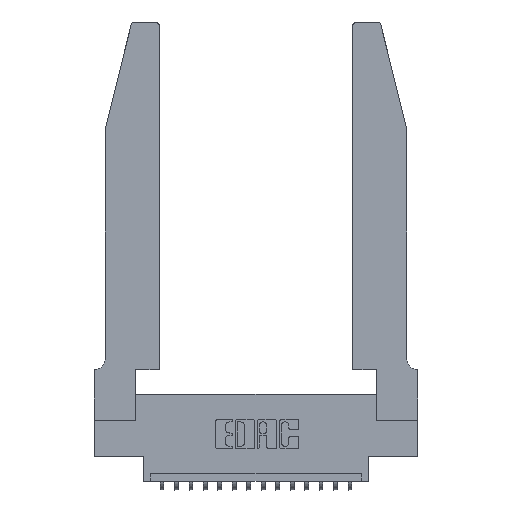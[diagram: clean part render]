
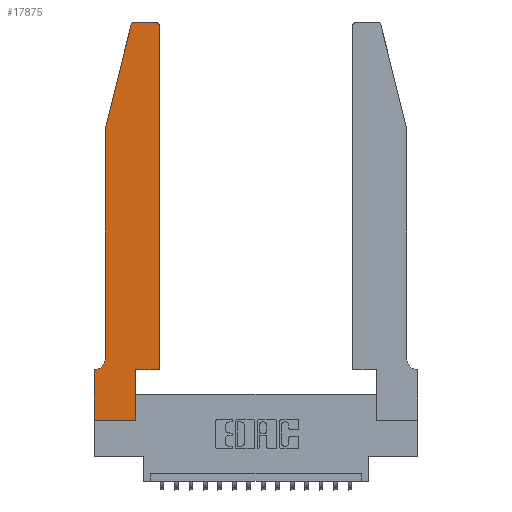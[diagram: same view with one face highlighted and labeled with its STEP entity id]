
A CAD part, top view. The second image highlights one B-rep face of the part: STEP entity #17875.
In plain terms, the highlighted planar face has unit normal (0, 0, 1).
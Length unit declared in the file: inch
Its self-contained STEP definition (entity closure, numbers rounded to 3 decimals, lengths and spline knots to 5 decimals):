
#250 = CARTESIAN_POINT ( 'NONE',  ( 0.0755, 0.35, 0.37 ) ) ;
#420 = CARTESIAN_POINT ( 'NONE',  ( 0.4505, 2.72, 0.37 ) ) ;
#478 = LINE ( 'NONE', #10517, #9352 ) ;
#524 = CARTESIAN_POINT ( 'NONE',  ( 0., 0.35, 0.37 ) ) ;
#538 = CARTESIAN_POINT ( 'NONE',  ( 0.25487, 2.72718, 0.37 ) ) ;
#930 = CARTESIAN_POINT ( 'NONE',  ( 0.0755, 2., 0.37 ) ) ;
#1041 = VECTOR ( 'NONE', #11612, 39.37008 ) ;
#2161 = CARTESIAN_POINT ( 'NONE',  ( 0.0755, 0.42, 0.37 ) ) ;
#2269 = DIRECTION ( 'NONE',  ( 1., 0., 0. ) ) ;
#2365 = EDGE_LOOP ( 'NONE', ( #7171, #6039, #3279, #11034, #11916, #15644, #4440, #10279, #8576, #5864, #8423, #12303 ) ) ;
#2465 = LINE ( 'NONE', #15607, #2705 ) ;
#2705 = VECTOR ( 'NONE', #3567, 39.37008 ) ;
#2795 = LINE ( 'NONE', #14105, #6289 ) ;
#3279 = ORIENTED_EDGE ( 'NONE', *, *, #13928, .T. ) ;
#3567 = DIRECTION ( 'NONE',  ( 1., 0., 0. ) ) ;
#3716 = VERTEX_POINT ( 'NONE', #5914 ) ;
#4440 = ORIENTED_EDGE ( 'NONE', *, *, #6249, .T. ) ;
#5052 = DIRECTION ( 'NONE',  ( 1., 0., 0. ) ) ;
#5201 = DIRECTION ( 'NONE',  ( 0., 0., -1. ) ) ;
#5593 = VERTEX_POINT ( 'NONE', #18524 ) ;
#5864 = ORIENTED_EDGE ( 'NONE', *, *, #7411, .T. ) ;
#5914 = CARTESIAN_POINT ( 'NONE',  ( 0.2865, 0., 0.37 ) ) ;
#5917 = CIRCLE ( 'NONE', #7857, 0.07 ) ;
#5996 = EDGE_CURVE ( 'NONE', #3716, #10725, #478, .T. ) ;
#6039 = ORIENTED_EDGE ( 'NONE', *, *, #7348, .T. ) ;
#6249 = EDGE_CURVE ( 'NONE', #5593, #18419, #2795, .T. ) ;
#6289 = VECTOR ( 'NONE', #17297, 39.37008 ) ;
#6533 = LINE ( 'NONE', #250, #9564 ) ;
#6800 = DIRECTION ( 'NONE',  ( 1., 0., 0. ) ) ;
#7103 = VERTEX_POINT ( 'NONE', #2161 ) ;
#7171 = ORIENTED_EDGE ( 'NONE', *, *, #7546, .T. ) ;
#7348 = EDGE_CURVE ( 'NONE', #12134, #17519, #15580, .T. ) ;
#7411 = EDGE_CURVE ( 'NONE', #10725, #18413, #12380, .T. ) ;
#7546 = EDGE_CURVE ( 'NONE', #13530, #12134, #13526, .T. ) ;
#7550 = CARTESIAN_POINT ( 'NONE',  ( 0.2865, 0.35, 0.37 ) ) ;
#7667 = DIRECTION ( 'NONE',  ( 0., 1., 0. ) ) ;
#7857 = AXIS2_PLACEMENT_3D ( 'NONE', #15683, #5201, #8165 ) ;
#8165 = DIRECTION ( 'NONE',  ( -1., 0., 0. ) ) ;
#8423 = ORIENTED_EDGE ( 'NONE', *, *, #16150, .T. ) ;
#8576 = ORIENTED_EDGE ( 'NONE', *, *, #5996, .T. ) ;
#8690 = CARTESIAN_POINT ( 'NONE',  ( 0.0755, 2., 0.37 ) ) ;
#8800 = VECTOR ( 'NONE', #9985, 39.37008 ) ;
#8871 = EDGE_CURVE ( 'NONE', #15242, #7103, #11606, .T. ) ;
#9186 = DIRECTION ( 'NONE',  ( 1., 0., 0. ) ) ;
#9352 = VECTOR ( 'NONE', #7667, 39.37008 ) ;
#9481 = PLANE ( 'NONE',  #9711 ) ;
#9564 = VECTOR ( 'NONE', #14778, 39.37008 ) ;
#9711 = AXIS2_PLACEMENT_3D ( 'NONE', #524, #12338, #5052 ) ;
#9985 = DIRECTION ( 'NONE',  ( 0., -1., 0. ) ) ;
#10125 = CIRCLE ( 'NONE', #16371, 0.03 ) ;
#10279 = ORIENTED_EDGE ( 'NONE', *, *, #15847, .T. ) ;
#10294 = CARTESIAN_POINT ( 'NONE',  ( 0.4505, 0.35, 0.37 ) ) ;
#10472 = VECTOR ( 'NONE', #13755, 39.37008 ) ;
#10517 = CARTESIAN_POINT ( 'NONE',  ( 0.2865, 0.35, 0.37 ) ) ;
#10654 = EDGE_CURVE ( 'NONE', #15326, #5593, #6533, .T. ) ;
#10725 = VERTEX_POINT ( 'NONE', #7550 ) ;
#11034 = ORIENTED_EDGE ( 'NONE', *, *, #8871, .T. ) ;
#11117 = CARTESIAN_POINT ( 'NONE',  ( 0., 0., 0.37 ) ) ;
#11606 = LINE ( 'NONE', #930, #8800 ) ;
#11612 = DIRECTION ( 'NONE',  ( 0., 1., 0. ) ) ;
#11682 = VECTOR ( 'NONE', #14471, 39.37008 ) ;
#11916 = ORIENTED_EDGE ( 'NONE', *, *, #17444, .T. ) ;
#12134 = VERTEX_POINT ( 'NONE', #17369 ) ;
#12299 = EDGE_CURVE ( 'NONE', #15215, #13530, #10125, .T. ) ;
#12303 = ORIENTED_EDGE ( 'NONE', *, *, #12299, .T. ) ;
#12338 = DIRECTION ( 'NONE',  ( 0., 0., 1. ) ) ;
#12380 = LINE ( 'NONE', #14260, #16733 ) ;
#12615 = LINE ( 'NONE', #8690, #11682 ) ;
#12993 = LINE ( 'NONE', #10294, #1041 ) ;
#13510 = DIRECTION ( 'NONE',  ( 0., 0., 1. ) ) ;
#13526 = LINE ( 'NONE', #18059, #10472 ) ;
#13530 = VERTEX_POINT ( 'NONE', #15190 ) ;
#13755 = DIRECTION ( 'NONE',  ( -1., 0., 0. ) ) ;
#13782 = CARTESIAN_POINT ( 'NONE',  ( 0.284, 2.72, 0.37 ) ) ;
#13928 = EDGE_CURVE ( 'NONE', #17519, #15242, #12615, .T. ) ;
#14105 = CARTESIAN_POINT ( 'NONE',  ( 0., 0., 0.37 ) ) ;
#14260 = CARTESIAN_POINT ( 'NONE',  ( 0.4505, 0.35, 0.37 ) ) ;
#14471 = DIRECTION ( 'NONE',  ( -0.239, -0.971, 0. ) ) ;
#14735 = AXIS2_PLACEMENT_3D ( 'NONE', #13782, #15560, #2269 ) ;
#14778 = DIRECTION ( 'NONE',  ( -1., 0., 0. ) ) ;
#14912 = CARTESIAN_POINT ( 'NONE',  ( 0.4205, 2.72, 0.37 ) ) ;
#15190 = CARTESIAN_POINT ( 'NONE',  ( 0.4205, 2.75, 0.37 ) ) ;
#15215 = VERTEX_POINT ( 'NONE', #420 ) ;
#15242 = VERTEX_POINT ( 'NONE', #18731 ) ;
#15326 = VERTEX_POINT ( 'NONE', #17123 ) ;
#15560 = DIRECTION ( 'NONE',  ( 0., 0., 1. ) ) ;
#15580 = CIRCLE ( 'NONE', #14735, 0.03 ) ;
#15607 = CARTESIAN_POINT ( 'NONE',  ( 0., 0., 0.37 ) ) ;
#15644 = ORIENTED_EDGE ( 'NONE', *, *, #10654, .T. ) ;
#15683 = CARTESIAN_POINT ( 'NONE',  ( 0.0055, 0.42, 0.37 ) ) ;
#15847 = EDGE_CURVE ( 'NONE', #18419, #3716, #2465, .T. ) ;
#16150 = EDGE_CURVE ( 'NONE', #18413, #15215, #12993, .T. ) ;
#16371 = AXIS2_PLACEMENT_3D ( 'NONE', #14912, #13510, #9186 ) ;
#16733 = VECTOR ( 'NONE', #6800, 39.37008 ) ;
#17123 = CARTESIAN_POINT ( 'NONE',  ( 0.0055, 0.35, 0.37 ) ) ;
#17297 = DIRECTION ( 'NONE',  ( 0., -1., 0. ) ) ;
#17369 = CARTESIAN_POINT ( 'NONE',  ( 0.284, 2.75, 0.37 ) ) ;
#17383 = FACE_OUTER_BOUND ( 'NONE', #2365, .T. ) ;
#17444 = EDGE_CURVE ( 'NONE', #7103, #15326, #5917, .T. ) ;
#17519 = VERTEX_POINT ( 'NONE', #538 ) ;
#17875 = ADVANCED_FACE ( 'NONE', ( #17383 ), #9481, .T. ) ;
#18059 = CARTESIAN_POINT ( 'NONE',  ( 0.2605, 2.75, 0.37 ) ) ;
#18296 = CARTESIAN_POINT ( 'NONE',  ( 0.4505, 0.35, 0.37 ) ) ;
#18413 = VERTEX_POINT ( 'NONE', #18296 ) ;
#18419 = VERTEX_POINT ( 'NONE', #11117 ) ;
#18524 = CARTESIAN_POINT ( 'NONE',  ( 0., 0.35, 0.37 ) ) ;
#18731 = CARTESIAN_POINT ( 'NONE',  ( 0.0755, 2., 0.37 ) ) ;
